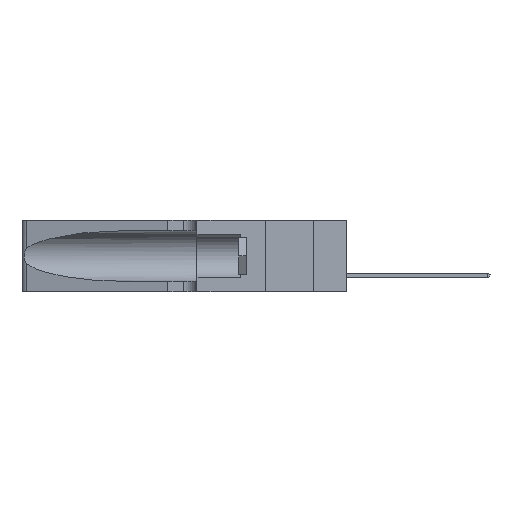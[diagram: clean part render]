
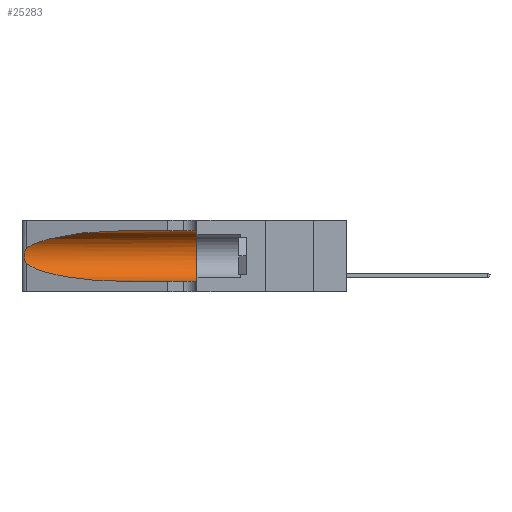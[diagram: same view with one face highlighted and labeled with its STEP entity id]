
A CAD part, left-side view. The second image highlights one B-rep face of the part: STEP entity #25283.
In plain terms, the highlighted cylindrical face has radius 3.308 mm (diameter 6.617 mm), a partial arc.
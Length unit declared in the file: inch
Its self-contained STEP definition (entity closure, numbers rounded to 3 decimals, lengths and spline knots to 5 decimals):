
#1697 = ORIENTED_EDGE ( 'NONE', *, *, #39376, .T. ) ;
#3829 = DIRECTION ( 'NONE',  ( 0., 0., -1. ) ) ;
#4191 = CARTESIAN_POINT ( 'NONE',  ( 0.1305, 1.61858, 0.31525 ) ) ;
#4837 = CARTESIAN_POINT ( 'NONE',  ( 0.1305, 0.35, 0.05475 ) ) ;
#4901 = CARTESIAN_POINT ( 'NONE',  ( 0.1305, 1.61858, 0.05475 ) ) ;
#5008 = CARTESIAN_POINT ( 'NONE',  ( 0.25555, 1.22994, 0.2215 ) ) ;
#5061 = DIRECTION ( 'NONE',  ( 0., -1., 0. ) ) ;
#5179 = CARTESIAN_POINT ( 'NONE',  ( 0.25787, 1.23484, 0.2124 ) ) ;
#5989 = VECTOR ( 'NONE', #5061, 39.37008 ) ;
#6188 = EDGE_LOOP ( 'NONE', ( #42439, #21387, #34946, #1697, #24012, #18048 ) ) ;
#9313 = CARTESIAN_POINT ( 'NONE',  ( 0.26017, 1.23833, 0.17102 ) ) ;
#9784 = CARTESIAN_POINT ( 'NONE',  ( 0.1305, 0.72297, 0.31525 ) ) ;
#10086 = DIRECTION ( 'NONE',  ( 0., -1., 0. ) ) ;
#11697 = VERTEX_POINT ( 'NONE', #31106 ) ;
#13206 = CARTESIAN_POINT ( 'NONE',  ( 0.18966, 0.96281, 0.05475 ) ) ;
#13942 = CARTESIAN_POINT ( 'NONE',  ( 0.25487, 1.22718, 0.14631 ) ) ;
#14406 = CARTESIAN_POINT ( 'NONE',  ( 0.1305, 0.72297, 0.05475 ) ) ;
#15048 = EDGE_CURVE ( 'NONE', #41224, #11697, #17039, .T. ) ;
#15585 = LINE ( 'NONE', #4901, #5989 ) ;
#16108 = CARTESIAN_POINT ( 'NONE',  ( 0.25854, 1.2359, 0.20912 ) ) ;
#16445 = CARTESIAN_POINT ( 'NONE',  ( 0.25789, 1.23486, 0.15765 ) ) ;
#16805 = CARTESIAN_POINT ( 'NONE',  ( 0.18966, 0.96281, 0.31525 ) ) ;
#17039 = B_SPLINE_CURVE_WITH_KNOTS ( 'NONE', 3,
 ( #37619, #5008, #30361, #5179, #16108, #18960, #45734, #45078, #9313, #37973, #16445, #38293, #42746, #13942 ),
 .UNSPECIFIED., .F., .F.,
 ( 4, 2, 2, 2, 2, 2, 4 ),
 ( 0., 0.00027, 0.00053, 0.00107, 0.0016, 0.00187, 0.00214 ),
 .UNSPECIFIED. ) ;
#18048 = ORIENTED_EDGE ( 'NONE', *, *, #23537, .F. ) ;
#18069 = CARTESIAN_POINT ( 'NONE',  ( 0.25487, 1.22718, 0.22369 ) ) ;
#18437 = CARTESIAN_POINT ( 'NONE',  ( 0.1305, 0.35, 0.31525 ) ) ;
#18520 = FACE_OUTER_BOUND ( 'NONE', #6188, .T. ) ;
#18960 = CARTESIAN_POINT ( 'NONE',  ( 0.26018, 1.23835, 0.19895 ) ) ;
#19323 = EDGE_CURVE ( 'NONE', #11697, #31836, #21378, .T. ) ;
#20437 = LINE ( 'NONE', #4191, #25474 ) ;
#21378 =( BOUNDED_CURVE ( )  B_SPLINE_CURVE ( 3, ( #45337, #26760, #13206, #14406 ),
 .UNSPECIFIED., .F., .T. ) 
 B_SPLINE_CURVE_WITH_KNOTS ( ( 4, 4 ),
 ( 3.44316, 4.71239 ),
 .UNSPECIFIED. ) 
 CURVE ( )  GEOMETRIC_REPRESENTATION_ITEM ( )  RATIONAL_B_SPLINE_CURVE ( ( 1., 0.87, 0.87, 1. ) ) 
 REPRESENTATION_ITEM ( '' )  );
#21387 = ORIENTED_EDGE ( 'NONE', *, *, #15048, .T. ) ;
#22018 = CARTESIAN_POINT ( 'NONE',  ( 0.1305, 0.72297, 0.31525 ) ) ;
#22593 = CARTESIAN_POINT ( 'NONE',  ( 0.1305, 0.72297, 0.05475 ) ) ;
#23055 = CARTESIAN_POINT ( 'NONE',  ( 0.1305, 0.35, 0.185 ) ) ;
#23332 = AXIS2_PLACEMENT_3D ( 'NONE', #23055, #45464, #30578 ) ;
#23537 = EDGE_CURVE ( 'NONE', #45015, #43126, #20437, .T. ) ;
#24012 = ORIENTED_EDGE ( 'NONE', *, *, #42266, .F. ) ;
#24166 = CARTESIAN_POINT ( 'NONE',  ( 0.1305, 1.61858, 0.185 ) ) ;
#25283 = ADVANCED_FACE ( 'NONE', ( #18520 ), #28774, .F. ) ;
#25474 = VECTOR ( 'NONE', #45055, 39.37008 ) ;
#26760 = CARTESIAN_POINT ( 'NONE',  ( 0.2373, 1.15595, 0.08982 ) ) ;
#27759 = CARTESIAN_POINT ( 'NONE',  ( 0.25487, 1.22718, 0.22369 ) ) ;
#27896 = EDGE_CURVE ( 'NONE', #45015, #41224, #38813, .T. ) ;
#28774 = CYLINDRICAL_SURFACE ( 'NONE', #32457, 0.13025 ) ;
#30361 = CARTESIAN_POINT ( 'NONE',  ( 0.25639, 1.23184, 0.21858 ) ) ;
#30578 = DIRECTION ( 'NONE',  ( 0., 0., 1. ) ) ;
#31106 = CARTESIAN_POINT ( 'NONE',  ( 0.25487, 1.22718, 0.14631 ) ) ;
#31836 = VERTEX_POINT ( 'NONE', #22593 ) ;
#32457 = AXIS2_PLACEMENT_3D ( 'NONE', #24166, #10086, #3829 ) ;
#34946 = ORIENTED_EDGE ( 'NONE', *, *, #19323, .T. ) ;
#37619 = CARTESIAN_POINT ( 'NONE',  ( 0.25487, 1.22718, 0.22369 ) ) ;
#37973 = CARTESIAN_POINT ( 'NONE',  ( 0.25856, 1.23593, 0.16098 ) ) ;
#38293 = CARTESIAN_POINT ( 'NONE',  ( 0.25639, 1.23186, 0.15144 ) ) ;
#38813 =( BOUNDED_CURVE ( )  B_SPLINE_CURVE ( 3, ( #22018, #16805, #42307, #18069 ),
 .UNSPECIFIED., .F., .F. ) 
 B_SPLINE_CURVE_WITH_KNOTS ( ( 4, 4 ),
 ( 1.5708, 2.84003 ),
 .UNSPECIFIED. ) 
 CURVE ( )  GEOMETRIC_REPRESENTATION_ITEM ( )  RATIONAL_B_SPLINE_CURVE ( ( 1., 0.87, 0.87, 1. ) ) 
 REPRESENTATION_ITEM ( '' )  );
#39376 = EDGE_CURVE ( 'NONE', #31836, #44710, #15585, .T. ) ;
#39897 = CIRCLE ( 'NONE', #23332, 0.13025 ) ;
#41224 = VERTEX_POINT ( 'NONE', #27759 ) ;
#42266 = EDGE_CURVE ( 'NONE', #43126, #44710, #39897, .T. ) ;
#42307 = CARTESIAN_POINT ( 'NONE',  ( 0.2373, 1.15595, 0.28018 ) ) ;
#42439 = ORIENTED_EDGE ( 'NONE', *, *, #27896, .T. ) ;
#42746 = CARTESIAN_POINT ( 'NONE',  ( 0.25555, 1.22993, 0.14849 ) ) ;
#43126 = VERTEX_POINT ( 'NONE', #18437 ) ;
#44710 = VERTEX_POINT ( 'NONE', #4837 ) ;
#45015 = VERTEX_POINT ( 'NONE', #9784 ) ;
#45055 = DIRECTION ( 'NONE',  ( 0., -1., 0. ) ) ;
#45078 = CARTESIAN_POINT ( 'NONE',  ( 0.26075, 1.23896, 0.178 ) ) ;
#45337 = CARTESIAN_POINT ( 'NONE',  ( 0.25487, 1.22718, 0.14631 ) ) ;
#45464 = DIRECTION ( 'NONE',  ( 0., 1., 0. ) ) ;
#45734 = CARTESIAN_POINT ( 'NONE',  ( 0.26075, 1.23896, 0.19203 ) ) ;
